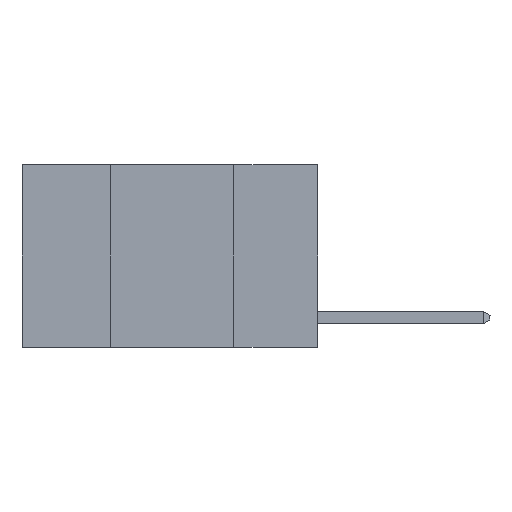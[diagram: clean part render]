
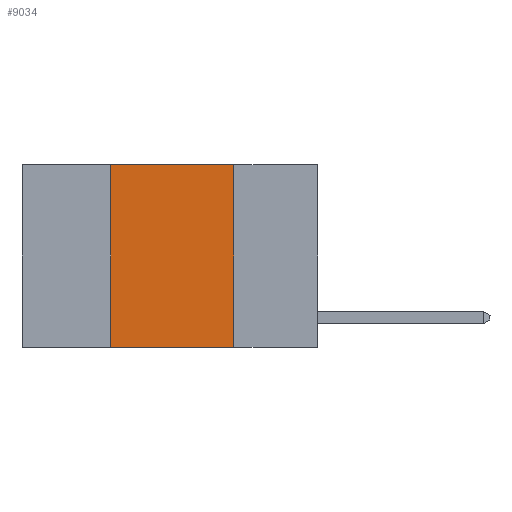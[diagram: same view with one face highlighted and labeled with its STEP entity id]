
A CAD part, left-side view. The second image highlights one B-rep face of the part: STEP entity #9034.
In plain terms, the highlighted planar face has unit normal (-1, 0, 0).
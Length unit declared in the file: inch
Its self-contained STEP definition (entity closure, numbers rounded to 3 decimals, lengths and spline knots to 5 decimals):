
#932 = ORIENTED_EDGE ( 'NONE', *, *, #18796, .F. ) ;
#3126 = CARTESIAN_POINT ( 'NONE',  ( 0., 0.6, 0. ) ) ;
#3464 = DIRECTION ( 'NONE',  ( 0., -1., 0. ) ) ;
#4059 = CARTESIAN_POINT ( 'NONE',  ( 0., 0.42, 0. ) ) ;
#5084 = CARTESIAN_POINT ( 'NONE',  ( 0., 0.17, 0. ) ) ;
#5397 = VECTOR ( 'NONE', #23832, 39.37008 ) ;
#5545 = VECTOR ( 'NONE', #3464, 39.37008 ) ;
#5595 = DIRECTION ( 'NONE',  ( 1., 0., 0. ) ) ;
#5795 = CARTESIAN_POINT ( 'NONE',  ( 0., 0.17, -0.37 ) ) ;
#7108 = AXIS2_PLACEMENT_3D ( 'NONE', #3126, #5595, #7913 ) ;
#7176 = LINE ( 'NONE', #7325, #5397 ) ;
#7186 = VECTOR ( 'NONE', #28546, 39.37008 ) ;
#7325 = CARTESIAN_POINT ( 'NONE',  ( 0., 0.42, 0. ) ) ;
#7630 = EDGE_CURVE ( 'NONE', #8113, #27607, #15202, .T. ) ;
#7913 = DIRECTION ( 'NONE',  ( 0., 0., -1. ) ) ;
#8063 = FACE_OUTER_BOUND ( 'NONE', #26399, .T. ) ;
#8113 = VERTEX_POINT ( 'NONE', #19781 ) ;
#9034 = ADVANCED_FACE ( 'NONE', ( #8063 ), #17331, .F. ) ;
#9697 = LINE ( 'NONE', #28549, #29581 ) ;
#9849 = CARTESIAN_POINT ( 'NONE',  ( 0., 0.17, 0. ) ) ;
#10057 = VERTEX_POINT ( 'NONE', #4059 ) ;
#15061 = CARTESIAN_POINT ( 'NONE',  ( 0., 0.6, -0.37 ) ) ;
#15202 = LINE ( 'NONE', #15061, #5545 ) ;
#16062 = DIRECTION ( 'NONE',  ( 0., -1., 0. ) ) ;
#17331 = PLANE ( 'NONE',  #7108 ) ;
#18474 = EDGE_CURVE ( 'NONE', #10057, #25790, #9697, .T. ) ;
#18796 = EDGE_CURVE ( 'NONE', #8113, #10057, #7176, .T. ) ;
#19406 = LINE ( 'NONE', #9849, #7186 ) ;
#19781 = CARTESIAN_POINT ( 'NONE',  ( 0., 0.42, -0.37 ) ) ;
#20580 = ORIENTED_EDGE ( 'NONE', *, *, #7630, .T. ) ;
#22140 = ORIENTED_EDGE ( 'NONE', *, *, #18474, .F. ) ;
#23832 = DIRECTION ( 'NONE',  ( 0., 0., 1. ) ) ;
#25790 = VERTEX_POINT ( 'NONE', #5084 ) ;
#26399 = EDGE_LOOP ( 'NONE', ( #28119, #22140, #932, #20580 ) ) ;
#26950 = EDGE_CURVE ( 'NONE', #25790, #27607, #19406, .T. ) ;
#27607 = VERTEX_POINT ( 'NONE', #5795 ) ;
#28119 = ORIENTED_EDGE ( 'NONE', *, *, #26950, .F. ) ;
#28546 = DIRECTION ( 'NONE',  ( 0., 0., -1. ) ) ;
#28549 = CARTESIAN_POINT ( 'NONE',  ( 0., 0.6, 0. ) ) ;
#29581 = VECTOR ( 'NONE', #16062, 39.37008 ) ;
